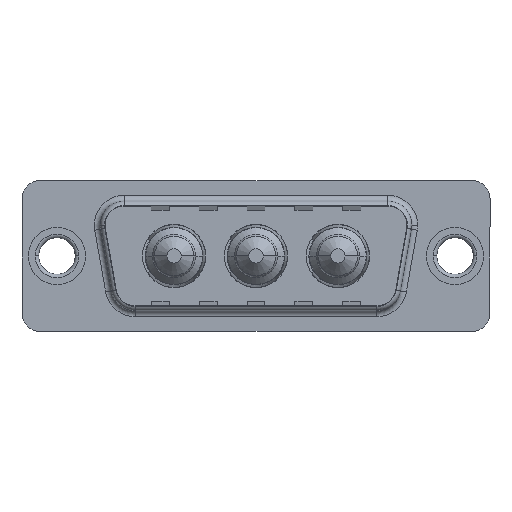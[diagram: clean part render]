
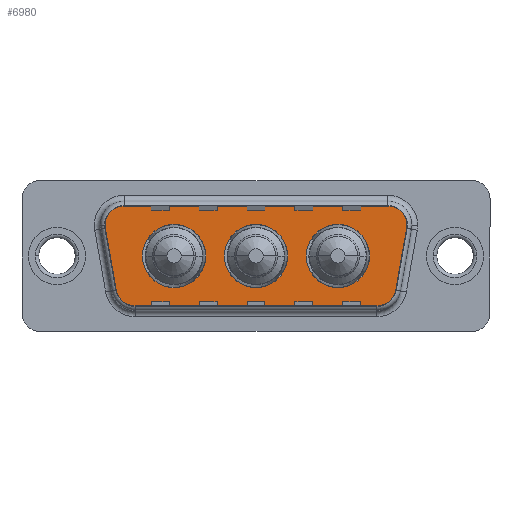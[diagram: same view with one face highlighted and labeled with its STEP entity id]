
A CAD part, top view. The second image highlights one B-rep face of the part: STEP entity #6980.
In plain terms, the highlighted planar face has unit normal (0, 0, 1).
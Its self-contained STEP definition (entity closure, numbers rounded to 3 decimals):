
#56 = DIRECTION ( 'NONE',  ( 0., 0., 1. ) ) ;
#61 = CARTESIAN_POINT ( 'NONE',  ( 23.5, 0., 0. ) ) ;
#104 = ORIENTED_EDGE ( 'NONE', *, *, #5111, .F. ) ;
#137 = DIRECTION ( 'NONE',  ( 1., 0., 0. ) ) ;
#214 = VERTEX_POINT ( 'NONE', #10971 ) ;
#346 = VERTEX_POINT ( 'NONE', #813 ) ;
#350 = DIRECTION ( 'NONE',  ( 0., 0., 1. ) ) ;
#373 = VECTOR ( 'NONE', #8208, 1000. ) ;
#457 = EDGE_CURVE ( 'NONE', #3707, #1165, #8908, .T. ) ;
#477 = VERTEX_POINT ( 'NONE', #3359 ) ;
#478 = EDGE_CURVE ( 'NONE', #5864, #8212, #1484, .T. ) ;
#587 = ORIENTED_EDGE ( 'NONE', *, *, #7321, .T. ) ;
#699 = ORIENTED_EDGE ( 'NONE', *, *, #8949, .T. ) ;
#813 = CARTESIAN_POINT ( 'NONE',  ( 28.836, -3.247, 0. ) ) ;
#824 = EDGE_LOOP ( 'NONE', ( #104, #5255 ) ) ;
#943 = DIRECTION ( 'NONE',  ( 1., 0., 0. ) ) ;
#949 = CIRCLE ( 'NONE', #8452, 2.65 ) ;
#1027 = AXIS2_PLACEMENT_3D ( 'NONE', #61, #6097, #943 ) ;
#1165 = VERTEX_POINT ( 'NONE', #6582 ) ;
#1260 = DIRECTION ( 'NONE',  ( -1., 0., 0. ) ) ;
#1369 = CARTESIAN_POINT ( 'NONE',  ( 9.8, 0., 0. ) ) ;
#1410 = ORIENTED_EDGE ( 'NONE', *, *, #457, .T. ) ;
#1417 = DIRECTION ( 'NONE',  ( 0., 0., 1. ) ) ;
#1484 = CIRCLE ( 'NONE', #7788, 2.65 ) ;
#1944 = CARTESIAN_POINT ( 'NONE',  ( 26.866, -2.9, 0. ) ) ;
#2160 = DIRECTION ( 'NONE',  ( 0.174, 0.985, 0. ) ) ;
#2190 = EDGE_CURVE ( 'NONE', #1165, #6265, #3113, .T. ) ;
#2342 = CARTESIAN_POINT ( 'NONE',  ( 26.15, 0., 0. ) ) ;
#2424 = ORIENTED_EDGE ( 'NONE', *, *, #9929, .T. ) ;
#2425 = EDGE_CURVE ( 'NONE', #8510, #9173, #2971, .T. ) ;
#2670 = FACE_BOUND ( 'NONE', #3220, .T. ) ;
#2723 = CARTESIAN_POINT ( 'NONE',  ( 6.434, -4.9, 0. ) ) ;
#2748 = CARTESIAN_POINT ( 'NONE',  ( 23.5, 0., 0. ) ) ;
#2834 = ORIENTED_EDGE ( 'NONE', *, *, #2190, .T. ) ;
#2839 = DIRECTION ( 'NONE',  ( 1., 0., 0. ) ) ;
#2865 = CIRCLE ( 'NONE', #10407, 2. ) ;
#2887 = CIRCLE ( 'NONE', #3573, 2. ) ;
#2889 = EDGE_CURVE ( 'NONE', #346, #8632, #6719, .T. ) ;
#2917 = AXIS2_PLACEMENT_3D ( 'NONE', #3934, #56, #4682 ) ;
#2931 = FACE_BOUND ( 'NONE', #4809, .T. ) ;
#2971 = LINE ( 'NONE', #8513, #373 ) ;
#3113 = LINE ( 'NONE', #4978, #4324 ) ;
#3117 = AXIS2_PLACEMENT_3D ( 'NONE', #2748, #6502, #137 ) ;
#3161 = VERTEX_POINT ( 'NONE', #7684 ) ;
#3220 = EDGE_LOOP ( 'NONE', ( #8249, #7715 ) ) ;
#3242 = CARTESIAN_POINT ( 'NONE',  ( 16.65, 0., 0. ) ) ;
#3359 = CARTESIAN_POINT ( 'NONE',  ( 27.889, 4.9, 0. ) ) ;
#3573 = AXIS2_PLACEMENT_3D ( 'NONE', #6591, #1417, #7447 ) ;
#3707 = VERTEX_POINT ( 'NONE', #9714 ) ;
#3743 = DIRECTION ( 'NONE',  ( 0., 0., 1. ) ) ;
#3838 = CIRCLE ( 'NONE', #7219, 2.65 ) ;
#3934 = CARTESIAN_POINT ( 'NONE',  ( 26.866, -2.9, 0. ) ) ;
#3940 = PLANE ( 'NONE',  #2917 ) ;
#3956 = VERTEX_POINT ( 'NONE', #2342 ) ;
#4223 = VERTEX_POINT ( 'NONE', #9962 ) ;
#4324 = VECTOR ( 'NONE', #4724, 1000. ) ;
#4428 = AXIS2_PLACEMENT_3D ( 'NONE', #5265, #8237, #10278 ) ;
#4515 = DIRECTION ( 'NONE',  ( -1., 0., 0. ) ) ;
#4558 = EDGE_CURVE ( 'NONE', #3956, #214, #7598, .T. ) ;
#4618 = ORIENTED_EDGE ( 'NONE', *, *, #2889, .T. ) ;
#4672 = CIRCLE ( 'NONE', #9297, 2. ) ;
#4682 = DIRECTION ( 'NONE',  ( 1., 0., 0. ) ) ;
#4718 = CARTESIAN_POINT ( 'NONE',  ( 5.411, 4.9, 0. ) ) ;
#4724 = DIRECTION ( 'NONE',  ( 0.174, -0.985, 0. ) ) ;
#4726 = DIRECTION ( 'NONE',  ( 0., 0., 1. ) ) ;
#4778 = VERTEX_POINT ( 'NONE', #6790 ) ;
#4809 = EDGE_LOOP ( 'NONE', ( #8534, #5646 ) ) ;
#4934 = FACE_OUTER_BOUND ( 'NONE', #10739, .T. ) ;
#4956 = DIRECTION ( 'NONE',  ( 0., 0., 1. ) ) ;
#4978 = CARTESIAN_POINT ( 'NONE',  ( 3.441, 2.553, 0. ) ) ;
#5111 = EDGE_CURVE ( 'NONE', #4778, #3161, #6802, .T. ) ;
#5221 = CARTESIAN_POINT ( 'NONE',  ( 29.859, 2.553, 0. ) ) ;
#5255 = ORIENTED_EDGE ( 'NONE', *, *, #5948, .F. ) ;
#5265 = CARTESIAN_POINT ( 'NONE',  ( 9.8, 0., 0. ) ) ;
#5508 = VECTOR ( 'NONE', #1260, 1000. ) ;
#5646 = ORIENTED_EDGE ( 'NONE', *, *, #9252, .F. ) ;
#5655 = DIRECTION ( 'NONE',  ( 1., 0., 0. ) ) ;
#5773 = ORIENTED_EDGE ( 'NONE', *, *, #6318, .T. ) ;
#5784 = CARTESIAN_POINT ( 'NONE',  ( 29.859, 2.553, 0. ) ) ;
#5864 = VERTEX_POINT ( 'NONE', #10938 ) ;
#5948 = EDGE_CURVE ( 'NONE', #3161, #4778, #3838, .T. ) ;
#6063 = AXIS2_PLACEMENT_3D ( 'NONE', #6884, #350, #5655 ) ;
#6097 = DIRECTION ( 'NONE',  ( 0., 0., 1. ) ) ;
#6260 = CIRCLE ( 'NONE', #8496, 2. ) ;
#6265 = VERTEX_POINT ( 'NONE', #8792 ) ;
#6318 = EDGE_CURVE ( 'NONE', #8632, #4223, #4672, .T. ) ;
#6502 = DIRECTION ( 'NONE',  ( 0., 0., 1. ) ) ;
#6582 = CARTESIAN_POINT ( 'NONE',  ( 3.441, 2.553, 0. ) ) ;
#6591 = CARTESIAN_POINT ( 'NONE',  ( 6.434, -2.9, 0. ) ) ;
#6719 = LINE ( 'NONE', #5221, #8983 ) ;
#6790 = CARTESIAN_POINT ( 'NONE',  ( 12.45, 0., 0. ) ) ;
#6802 = CIRCLE ( 'NONE', #4428, 2.65 ) ;
#6884 = CARTESIAN_POINT ( 'NONE',  ( 5.411, 2.9, 0. ) ) ;
#6980 = ADVANCED_FACE ( 'NONE', ( #2670, #2931, #9511, #4934 ), #3940, .T. ) ;
#7219 = AXIS2_PLACEMENT_3D ( 'NONE', #1369, #4726, #9431 ) ;
#7321 = EDGE_CURVE ( 'NONE', #4223, #477, #6260, .T. ) ;
#7447 = DIRECTION ( 'NONE',  ( -1., 0., 0. ) ) ;
#7598 = CIRCLE ( 'NONE', #3117, 2.65 ) ;
#7684 = CARTESIAN_POINT ( 'NONE',  ( 7.15, 0., 0. ) ) ;
#7715 = ORIENTED_EDGE ( 'NONE', *, *, #10198, .F. ) ;
#7788 = AXIS2_PLACEMENT_3D ( 'NONE', #3242, #3743, #10942 ) ;
#7798 = LINE ( 'NONE', #4718, #5508 ) ;
#7838 = ORIENTED_EDGE ( 'NONE', *, *, #2425, .T. ) ;
#7969 = DIRECTION ( 'NONE',  ( 0., 0., 1. ) ) ;
#8123 = DIRECTION ( 'NONE',  ( -1., 0., 0. ) ) ;
#8175 = DIRECTION ( 'NONE',  ( 0., 0., 1. ) ) ;
#8198 = CARTESIAN_POINT ( 'NONE',  ( 27.889, 2.9, 0. ) ) ;
#8208 = DIRECTION ( 'NONE',  ( 1., 0., 0. ) ) ;
#8212 = VERTEX_POINT ( 'NONE', #8557 ) ;
#8237 = DIRECTION ( 'NONE',  ( 0., 0., 1. ) ) ;
#8249 = ORIENTED_EDGE ( 'NONE', *, *, #478, .F. ) ;
#8367 = DIRECTION ( 'NONE',  ( 0., 0., 1. ) ) ;
#8452 = AXIS2_PLACEMENT_3D ( 'NONE', #10095, #4956, #10981 ) ;
#8496 = AXIS2_PLACEMENT_3D ( 'NONE', #8198, #8175, #8123 ) ;
#8510 = VERTEX_POINT ( 'NONE', #2723 ) ;
#8513 = CARTESIAN_POINT ( 'NONE',  ( 6.434, -4.9, 0. ) ) ;
#8534 = ORIENTED_EDGE ( 'NONE', *, *, #4558, .F. ) ;
#8557 = CARTESIAN_POINT ( 'NONE',  ( 14., 0., 0. ) ) ;
#8632 = VERTEX_POINT ( 'NONE', #5784 ) ;
#8792 = CARTESIAN_POINT ( 'NONE',  ( 4.464, -3.247, 0. ) ) ;
#8908 = CIRCLE ( 'NONE', #6063, 2. ) ;
#8949 = EDGE_CURVE ( 'NONE', #6265, #8510, #2887, .T. ) ;
#8983 = VECTOR ( 'NONE', #2160, 1000. ) ;
#9173 = VERTEX_POINT ( 'NONE', #11158 ) ;
#9252 = EDGE_CURVE ( 'NONE', #214, #3956, #10805, .T. ) ;
#9266 = CARTESIAN_POINT ( 'NONE',  ( 27.889, 2.9, 0. ) ) ;
#9297 = AXIS2_PLACEMENT_3D ( 'NONE', #9266, #8367, #4515 ) ;
#9431 = DIRECTION ( 'NONE',  ( 1., 0., 0. ) ) ;
#9511 = FACE_BOUND ( 'NONE', #824, .T. ) ;
#9714 = CARTESIAN_POINT ( 'NONE',  ( 5.411, 4.9, 0. ) ) ;
#9929 = EDGE_CURVE ( 'NONE', #9173, #346, #2865, .T. ) ;
#9939 = ORIENTED_EDGE ( 'NONE', *, *, #11133, .T. ) ;
#9962 = CARTESIAN_POINT ( 'NONE',  ( 29.889, 2.9, 0. ) ) ;
#10095 = CARTESIAN_POINT ( 'NONE',  ( 16.65, 0., 0. ) ) ;
#10198 = EDGE_CURVE ( 'NONE', #8212, #5864, #949, .T. ) ;
#10278 = DIRECTION ( 'NONE',  ( 1., 0., 0. ) ) ;
#10407 = AXIS2_PLACEMENT_3D ( 'NONE', #1944, #7969, #2839 ) ;
#10739 = EDGE_LOOP ( 'NONE', ( #2424, #4618, #5773, #587, #9939, #1410, #2834, #699, #7838 ) ) ;
#10805 = CIRCLE ( 'NONE', #1027, 2.65 ) ;
#10938 = CARTESIAN_POINT ( 'NONE',  ( 19.3, 0., 0. ) ) ;
#10942 = DIRECTION ( 'NONE',  ( 1., 0., 0. ) ) ;
#10971 = CARTESIAN_POINT ( 'NONE',  ( 20.85, 0., 0. ) ) ;
#10981 = DIRECTION ( 'NONE',  ( 1., 0., 0. ) ) ;
#11133 = EDGE_CURVE ( 'NONE', #477, #3707, #7798, .T. ) ;
#11158 = CARTESIAN_POINT ( 'NONE',  ( 26.866, -4.9, 0. ) ) ;
